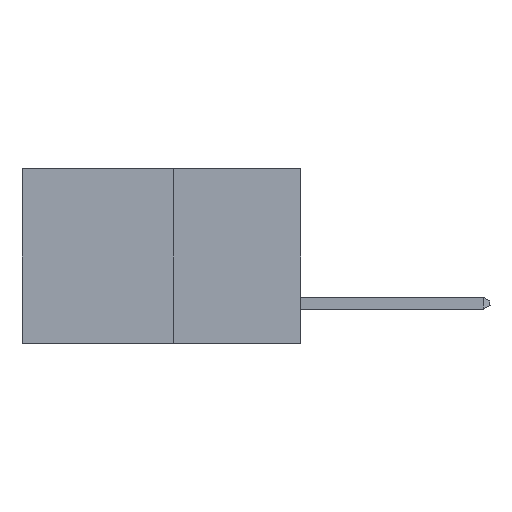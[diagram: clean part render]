
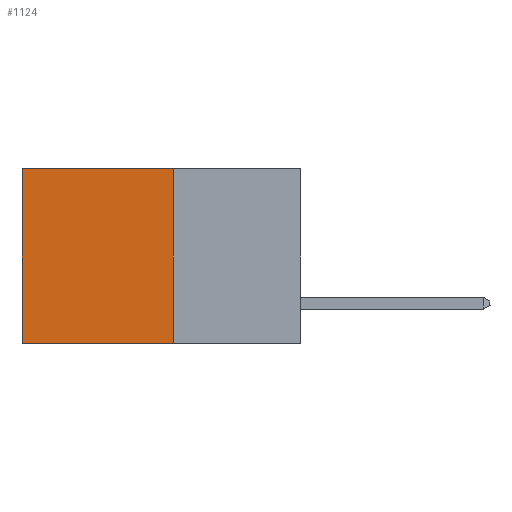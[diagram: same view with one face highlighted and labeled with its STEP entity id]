
A CAD part, left-side view. The second image highlights one B-rep face of the part: STEP entity #1124.
In plain terms, the highlighted planar face has unit normal (-1, 0, 0).
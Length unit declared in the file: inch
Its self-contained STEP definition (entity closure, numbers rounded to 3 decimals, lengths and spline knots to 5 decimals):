
#118 = PLANE ( 'NONE',  #18700 ) ;
#663 = CARTESIAN_POINT ( 'NONE',  ( 0.277, 0.27, 0. ) ) ;
#883 = EDGE_CURVE ( 'NONE', #17104, #18158, #6026, .T. ) ;
#1124 = ADVANCED_FACE ( 'NONE', ( #14178 ), #118, .F. ) ;
#1157 = CARTESIAN_POINT ( 'NONE',  ( 0.277, 0.27, 0. ) ) ;
#1237 = DIRECTION ( 'NONE',  ( 0., 1., 0. ) ) ;
#2932 = EDGE_LOOP ( 'NONE', ( #3867, #14836, #10892, #11423 ) ) ;
#3867 = ORIENTED_EDGE ( 'NONE', *, *, #883, .T. ) ;
#4693 = VECTOR ( 'NONE', #7094, 39.37008 ) ;
#5225 = VECTOR ( 'NONE', #20129, 39.37008 ) ;
#6026 = LINE ( 'NONE', #22938, #10258 ) ;
#6088 = LINE ( 'NONE', #1157, #9758 ) ;
#7094 = DIRECTION ( 'NONE',  ( 0., 1., 0. ) ) ;
#8026 = EDGE_CURVE ( 'NONE', #8212, #18158, #10085, .T. ) ;
#8212 = VERTEX_POINT ( 'NONE', #18189 ) ;
#9758 = VECTOR ( 'NONE', #1237, 39.37008 ) ;
#10085 = LINE ( 'NONE', #22998, #4693 ) ;
#10160 = EDGE_CURVE ( 'NONE', #11502, #8212, #19433, .T. ) ;
#10258 = VECTOR ( 'NONE', #22451, 39.37008 ) ;
#10892 = ORIENTED_EDGE ( 'NONE', *, *, #10160, .F. ) ;
#11017 = EDGE_CURVE ( 'NONE', #11502, #17104, #6088, .T. ) ;
#11423 = ORIENTED_EDGE ( 'NONE', *, *, #11017, .T. ) ;
#11502 = VERTEX_POINT ( 'NONE', #663 ) ;
#12562 = CARTESIAN_POINT ( 'NONE',  ( 0.277, 0.59, -0.37 ) ) ;
#14178 = FACE_OUTER_BOUND ( 'NONE', #2932, .T. ) ;
#14811 = CARTESIAN_POINT ( 'NONE',  ( 0.277, 0.59, 0. ) ) ;
#14836 = ORIENTED_EDGE ( 'NONE', *, *, #8026, .F. ) ;
#16239 = DIRECTION ( 'NONE',  ( 1., 0., 0. ) ) ;
#16267 = CARTESIAN_POINT ( 'NONE',  ( 0.277, 0.27, -0.37 ) ) ;
#17104 = VERTEX_POINT ( 'NONE', #14811 ) ;
#17863 = DIRECTION ( 'NONE',  ( 0., 0., -1. ) ) ;
#18158 = VERTEX_POINT ( 'NONE', #12562 ) ;
#18189 = CARTESIAN_POINT ( 'NONE',  ( 0.277, 0.27, -0.37 ) ) ;
#18344 = CARTESIAN_POINT ( 'NONE',  ( 0.277, 0.27, -0.37 ) ) ;
#18700 = AXIS2_PLACEMENT_3D ( 'NONE', #16267, #16239, #17863 ) ;
#19433 = LINE ( 'NONE', #18344, #5225 ) ;
#20129 = DIRECTION ( 'NONE',  ( 0., 0., -1. ) ) ;
#22451 = DIRECTION ( 'NONE',  ( 0., 0., -1. ) ) ;
#22938 = CARTESIAN_POINT ( 'NONE',  ( 0.277, 0.59, -0.37 ) ) ;
#22998 = CARTESIAN_POINT ( 'NONE',  ( 0.277, 0.27, -0.37 ) ) ;
